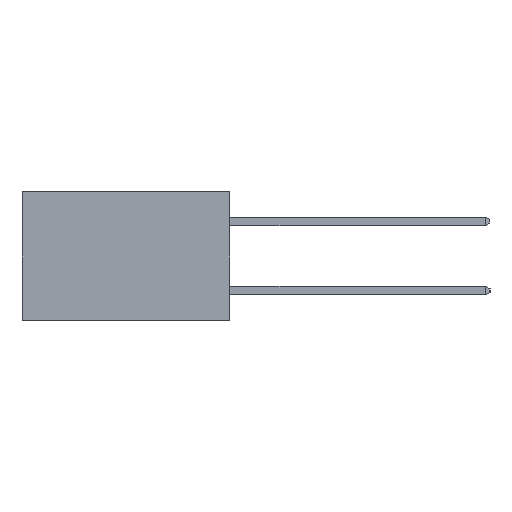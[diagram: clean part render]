
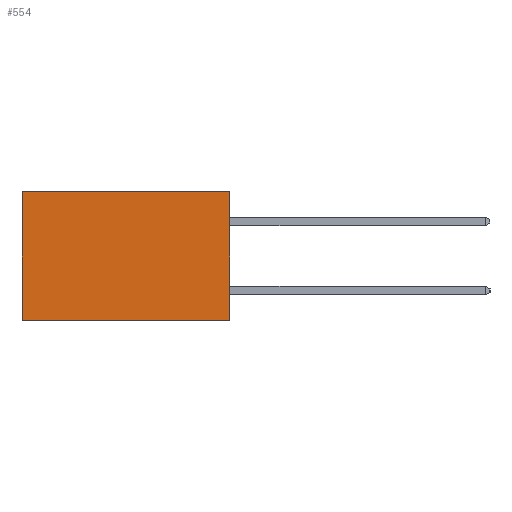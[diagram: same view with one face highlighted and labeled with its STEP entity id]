
A CAD part, left-side view. The second image highlights one B-rep face of the part: STEP entity #554.
In plain terms, the highlighted planar face has unit normal (-1, 0, 0).
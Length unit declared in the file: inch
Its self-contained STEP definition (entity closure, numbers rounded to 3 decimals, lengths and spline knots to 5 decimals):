
#510 = VECTOR ( 'NONE', #2645, 39.37008 ) ;
#544 = CARTESIAN_POINT ( 'NONE',  ( 0.2615, 0., 0. ) ) ;
#554 = ADVANCED_FACE ( 'NONE', ( #7205 ), #3228, .F. ) ;
#1069 = CARTESIAN_POINT ( 'NONE',  ( 0.2615, 0., 0. ) ) ;
#1468 = VERTEX_POINT ( 'NONE', #1069 ) ;
#1856 = EDGE_CURVE ( 'NONE', #7905, #2477, #8917, .T. ) ;
#1982 = EDGE_CURVE ( 'NONE', #1468, #7905, #3836, .T. ) ;
#2358 = DIRECTION ( 'NONE',  ( 0., 0., -1. ) ) ;
#2402 = CARTESIAN_POINT ( 'NONE',  ( 0.2615, 0., -0.37 ) ) ;
#2477 = VERTEX_POINT ( 'NONE', #7988 ) ;
#2487 = VECTOR ( 'NONE', #6275, 39.37008 ) ;
#2645 = DIRECTION ( 'NONE',  ( 0., 1., 0. ) ) ;
#3198 = CARTESIAN_POINT ( 'NONE',  ( 0.2615, 0.6, 0. ) ) ;
#3228 = PLANE ( 'NONE',  #3311 ) ;
#3311 = AXIS2_PLACEMENT_3D ( 'NONE', #15077, #5719, #5414 ) ;
#3836 = LINE ( 'NONE', #544, #510 ) ;
#4606 = ORIENTED_EDGE ( 'NONE', *, *, #14197, .F. ) ;
#4734 = EDGE_CURVE ( 'NONE', #1468, #6264, #5211, .T. ) ;
#5211 = LINE ( 'NONE', #2402, #11697 ) ;
#5414 = DIRECTION ( 'NONE',  ( 0., 0., -1. ) ) ;
#5719 = DIRECTION ( 'NONE',  ( 1., 0., 0. ) ) ;
#6227 = CARTESIAN_POINT ( 'NONE',  ( 0.2615, 0.6, -0.37 ) ) ;
#6264 = VERTEX_POINT ( 'NONE', #7791 ) ;
#6275 = DIRECTION ( 'NONE',  ( 0., 0., -1. ) ) ;
#7205 = FACE_OUTER_BOUND ( 'NONE', #12378, .T. ) ;
#7791 = CARTESIAN_POINT ( 'NONE',  ( 0.2615, 0., -0.37 ) ) ;
#7905 = VERTEX_POINT ( 'NONE', #3198 ) ;
#7988 = CARTESIAN_POINT ( 'NONE',  ( 0.2615, 0.6, -0.37 ) ) ;
#8917 = LINE ( 'NONE', #6227, #2487 ) ;
#9175 = LINE ( 'NONE', #13644, #15143 ) ;
#9344 = ORIENTED_EDGE ( 'NONE', *, *, #4734, .F. ) ;
#10752 = ORIENTED_EDGE ( 'NONE', *, *, #1982, .T. ) ;
#11697 = VECTOR ( 'NONE', #2358, 39.37008 ) ;
#12378 = EDGE_LOOP ( 'NONE', ( #13473, #4606, #9344, #10752 ) ) ;
#13473 = ORIENTED_EDGE ( 'NONE', *, *, #1856, .T. ) ;
#13644 = CARTESIAN_POINT ( 'NONE',  ( 0.2615, 0., -0.37 ) ) ;
#13693 = DIRECTION ( 'NONE',  ( 0., 1., 0. ) ) ;
#14197 = EDGE_CURVE ( 'NONE', #6264, #2477, #9175, .T. ) ;
#15077 = CARTESIAN_POINT ( 'NONE',  ( 0.2615, 0., -0.37 ) ) ;
#15143 = VECTOR ( 'NONE', #13693, 39.37008 ) ;
